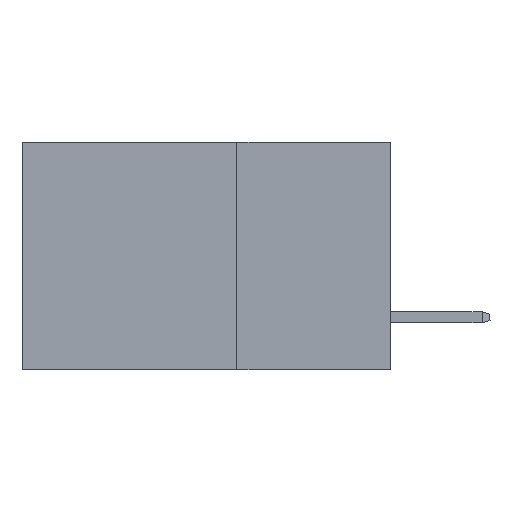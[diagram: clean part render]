
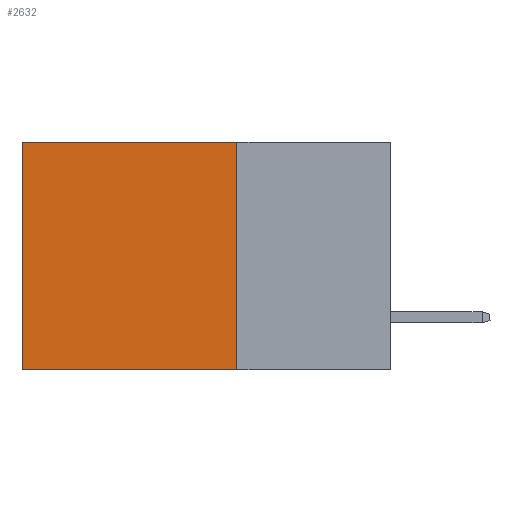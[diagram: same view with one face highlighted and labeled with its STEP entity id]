
A CAD part, left-side view. The second image highlights one B-rep face of the part: STEP entity #2632.
In plain terms, the highlighted planar face has unit normal (-1, 0, 0).
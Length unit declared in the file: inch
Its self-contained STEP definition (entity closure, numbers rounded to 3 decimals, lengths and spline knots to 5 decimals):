
#298 = ORIENTED_EDGE ( 'NONE', *, *, #7788, .T. ) ;
#315 = DIRECTION ( 'NONE',  ( 0., 0., -1. ) ) ;
#585 = LINE ( 'NONE', #10244, #6708 ) ;
#782 = VECTOR ( 'NONE', #7786, 39.37008 ) ;
#1595 = CARTESIAN_POINT ( 'NONE',  ( 0.2875, 0.6, 0. ) ) ;
#1928 = ORIENTED_EDGE ( 'NONE', *, *, #11934, .F. ) ;
#2501 = CARTESIAN_POINT ( 'NONE',  ( 0.2875, 0.25, 0. ) ) ;
#2632 = ADVANCED_FACE ( 'NONE', ( #11014 ), #9251, .F. ) ;
#3447 = LINE ( 'NONE', #2501, #782 ) ;
#3806 = DIRECTION ( 'NONE',  ( 0., 0., -1. ) ) ;
#4369 = CARTESIAN_POINT ( 'NONE',  ( 0.2875, 0.6, -0.37 ) ) ;
#4601 = DIRECTION ( 'NONE',  ( 1., 0., 0. ) ) ;
#4658 = LINE ( 'NONE', #1595, #8333 ) ;
#5462 = ORIENTED_EDGE ( 'NONE', *, *, #10739, .F. ) ;
#6708 = VECTOR ( 'NONE', #3806, 39.37008 ) ;
#7137 = EDGE_LOOP ( 'NONE', ( #298, #5462, #1928, #9631 ) ) ;
#7266 = CARTESIAN_POINT ( 'NONE',  ( 0.2875, 0.25, 0. ) ) ;
#7786 = DIRECTION ( 'NONE',  ( 0., 1., 0. ) ) ;
#7788 = EDGE_CURVE ( 'NONE', #12835, #11392, #4658, .T. ) ;
#7925 = VECTOR ( 'NONE', #8357, 39.37008 ) ;
#8333 = VECTOR ( 'NONE', #12244, 39.37008 ) ;
#8357 = DIRECTION ( 'NONE',  ( 0., 1., 0. ) ) ;
#8370 = AXIS2_PLACEMENT_3D ( 'NONE', #9957, #4601, #315 ) ;
#8860 = CARTESIAN_POINT ( 'NONE',  ( 0.2875, 0.6, 0. ) ) ;
#9251 = PLANE ( 'NONE',  #8370 ) ;
#9631 = ORIENTED_EDGE ( 'NONE', *, *, #10362, .T. ) ;
#9957 = CARTESIAN_POINT ( 'NONE',  ( 0.2875, 0.25, 0. ) ) ;
#10118 = LINE ( 'NONE', #12693, #7925 ) ;
#10244 = CARTESIAN_POINT ( 'NONE',  ( 0.2875, 0.25, 0. ) ) ;
#10362 = EDGE_CURVE ( 'NONE', #13684, #12835, #3447, .T. ) ;
#10739 = EDGE_CURVE ( 'NONE', #12883, #11392, #10118, .T. ) ;
#11014 = FACE_OUTER_BOUND ( 'NONE', #7137, .T. ) ;
#11154 = CARTESIAN_POINT ( 'NONE',  ( 0.2875, 0.25, -0.37 ) ) ;
#11392 = VERTEX_POINT ( 'NONE', #4369 ) ;
#11934 = EDGE_CURVE ( 'NONE', #13684, #12883, #585, .T. ) ;
#12244 = DIRECTION ( 'NONE',  ( 0., 0., -1. ) ) ;
#12693 = CARTESIAN_POINT ( 'NONE',  ( 0.2875, 0.25, -0.37 ) ) ;
#12835 = VERTEX_POINT ( 'NONE', #8860 ) ;
#12883 = VERTEX_POINT ( 'NONE', #11154 ) ;
#13684 = VERTEX_POINT ( 'NONE', #7266 ) ;
